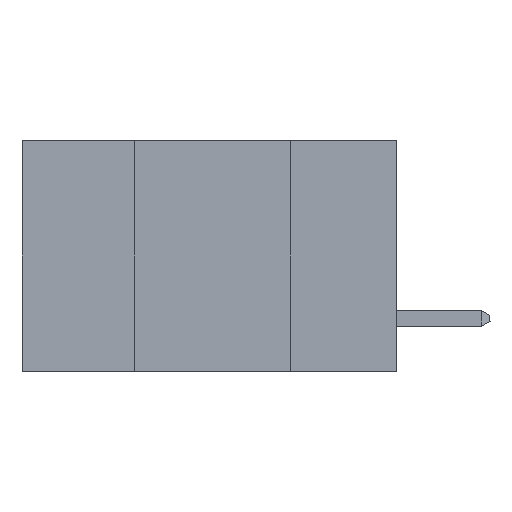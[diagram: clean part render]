
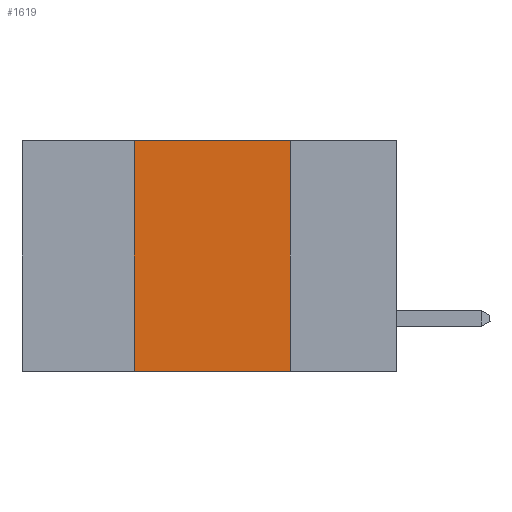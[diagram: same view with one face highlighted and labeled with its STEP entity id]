
A CAD part, left-side view. The second image highlights one B-rep face of the part: STEP entity #1619.
In plain terms, the highlighted planar face has unit normal (-1, 0, 0).
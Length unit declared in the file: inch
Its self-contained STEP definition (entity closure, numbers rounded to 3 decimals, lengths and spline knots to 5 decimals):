
#1016 = ORIENTED_EDGE ( 'NONE', *, *, #5779, .F. ) ;
#1190 = DIRECTION ( 'NONE',  ( 0., 0., -1. ) ) ;
#1200 = VECTOR ( 'NONE', #14882, 39.37008 ) ;
#1220 = EDGE_CURVE ( 'NONE', #7902, #13993, #7048, .T. ) ;
#1335 = LINE ( 'NONE', #7343, #8849 ) ;
#1430 = LINE ( 'NONE', #8000, #9404 ) ;
#1619 = ADVANCED_FACE ( 'NONE', ( #7473 ), #5561, .F. ) ;
#3828 = EDGE_LOOP ( 'NONE', ( #8054, #12472, #1016, #12915 ) ) ;
#4387 = CARTESIAN_POINT ( 'NONE',  ( 0., 0.17, -0.37 ) ) ;
#5335 = DIRECTION ( 'NONE',  ( 1., 0., 0. ) ) ;
#5545 = CARTESIAN_POINT ( 'NONE',  ( 0., 0.42, -0.37 ) ) ;
#5561 = PLANE ( 'NONE',  #6487 ) ;
#5779 = EDGE_CURVE ( 'NONE', #16759, #8540, #1335, .T. ) ;
#6487 = AXIS2_PLACEMENT_3D ( 'NONE', #10343, #5335, #1190 ) ;
#6673 = DIRECTION ( 'NONE',  ( 0., 0., 1. ) ) ;
#7048 = LINE ( 'NONE', #16775, #17798 ) ;
#7343 = CARTESIAN_POINT ( 'NONE',  ( 0., 0.42, 0. ) ) ;
#7473 = FACE_OUTER_BOUND ( 'NONE', #3828, .T. ) ;
#7902 = VERTEX_POINT ( 'NONE', #15860 ) ;
#8000 = CARTESIAN_POINT ( 'NONE',  ( 0., 0.6, -0.37 ) ) ;
#8054 = ORIENTED_EDGE ( 'NONE', *, *, #1220, .F. ) ;
#8540 = VERTEX_POINT ( 'NONE', #12883 ) ;
#8849 = VECTOR ( 'NONE', #6673, 39.37008 ) ;
#9404 = VECTOR ( 'NONE', #18214, 39.37008 ) ;
#9440 = EDGE_CURVE ( 'NONE', #8540, #7902, #16470, .T. ) ;
#9625 = EDGE_CURVE ( 'NONE', #16759, #13993, #1430, .T. ) ;
#10343 = CARTESIAN_POINT ( 'NONE',  ( 0., 0.6, 0. ) ) ;
#12472 = ORIENTED_EDGE ( 'NONE', *, *, #9440, .F. ) ;
#12883 = CARTESIAN_POINT ( 'NONE',  ( 0., 0.42, 0. ) ) ;
#12915 = ORIENTED_EDGE ( 'NONE', *, *, #9625, .T. ) ;
#13443 = CARTESIAN_POINT ( 'NONE',  ( 0., 0.6, 0. ) ) ;
#13993 = VERTEX_POINT ( 'NONE', #4387 ) ;
#14882 = DIRECTION ( 'NONE',  ( 0., -1., 0. ) ) ;
#15860 = CARTESIAN_POINT ( 'NONE',  ( 0., 0.17, 0. ) ) ;
#16470 = LINE ( 'NONE', #13443, #1200 ) ;
#16759 = VERTEX_POINT ( 'NONE', #5545 ) ;
#16775 = CARTESIAN_POINT ( 'NONE',  ( 0., 0.17, 0. ) ) ;
#16792 = DIRECTION ( 'NONE',  ( 0., 0., -1. ) ) ;
#17798 = VECTOR ( 'NONE', #16792, 39.37008 ) ;
#18214 = DIRECTION ( 'NONE',  ( 0., -1., 0. ) ) ;
